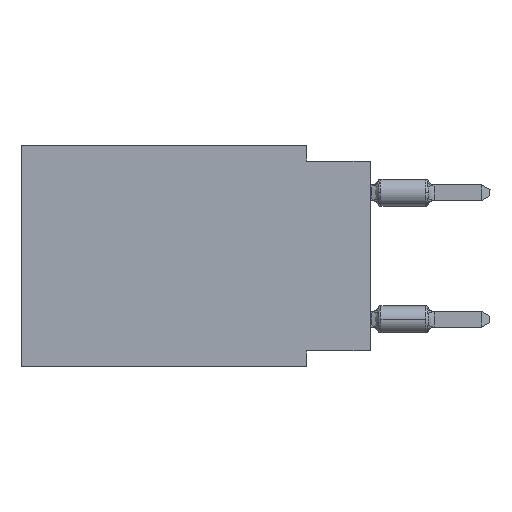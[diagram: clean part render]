
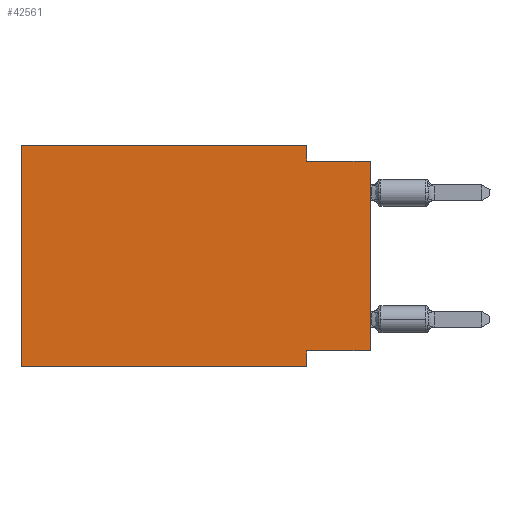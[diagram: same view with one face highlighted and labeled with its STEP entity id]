
A CAD part, left-side view. The second image highlights one B-rep face of the part: STEP entity #42561.
In plain terms, the highlighted planar face has unit normal (-1, 0, 0).
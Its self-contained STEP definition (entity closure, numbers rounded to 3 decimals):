
#1793 = VERTEX_POINT ( 'NONE', #42970 ) ;
#2512 = CARTESIAN_POINT ( 'NONE',  ( 0., 13.97, 0. ) ) ;
#2854 = VECTOR ( 'NONE', #18139, 1000. ) ;
#2898 = CARTESIAN_POINT ( 'NONE',  ( 0., 0., -8.255 ) ) ;
#2917 = EDGE_CURVE ( 'NONE', #43926, #25107, #45139, .T. ) ;
#3358 = CARTESIAN_POINT ( 'NONE',  ( 0., 2.54, 0. ) ) ;
#3403 = CARTESIAN_POINT ( 'NONE',  ( 0., 2.54, -8.89 ) ) ;
#4902 = EDGE_CURVE ( 'NONE', #26512, #8905, #33736, .T. ) ;
#6774 = CARTESIAN_POINT ( 'NONE',  ( 0., 0., -0.635 ) ) ;
#7037 = ORIENTED_EDGE ( 'NONE', *, *, #20022, .F. ) ;
#7201 = LINE ( 'NONE', #2512, #2854 ) ;
#8905 = VERTEX_POINT ( 'NONE', #49369 ) ;
#9450 = CARTESIAN_POINT ( 'NONE',  ( 0., 2.54, 0. ) ) ;
#10574 = LINE ( 'NONE', #26464, #40328 ) ;
#11358 = DIRECTION ( 'NONE',  ( 0., 0., -1. ) ) ;
#11938 = CARTESIAN_POINT ( 'NONE',  ( 0., 0., -0.635 ) ) ;
#12310 = ORIENTED_EDGE ( 'NONE', *, *, #32414, .T. ) ;
#12445 = LINE ( 'NONE', #11938, #13998 ) ;
#13086 = CARTESIAN_POINT ( 'NONE',  ( 0., 13.97, -8.89 ) ) ;
#13496 = VECTOR ( 'NONE', #34929, 1000. ) ;
#13998 = VECTOR ( 'NONE', #31977, 1000. ) ;
#14759 = EDGE_CURVE ( 'NONE', #8905, #43926, #7201, .T. ) ;
#14788 = VECTOR ( 'NONE', #29049, 1000. ) ;
#15261 = FACE_OUTER_BOUND ( 'NONE', #15369, .T. ) ;
#15296 = LINE ( 'NONE', #38744, #50191 ) ;
#15317 = ORIENTED_EDGE ( 'NONE', *, *, #14759, .F. ) ;
#15369 = EDGE_LOOP ( 'NONE', ( #43587, #40888, #17756, #15317, #21226, #12310, #7037, #40070 ) ) ;
#15669 = CARTESIAN_POINT ( 'NONE',  ( 0., 13.97, -8.89 ) ) ;
#17756 = ORIENTED_EDGE ( 'NONE', *, *, #2917, .F. ) ;
#17856 = CARTESIAN_POINT ( 'NONE',  ( 0., 13.97, 0. ) ) ;
#18139 = DIRECTION ( 'NONE',  ( 0., -1., 0. ) ) ;
#19164 = VECTOR ( 'NONE', #30226, 1000. ) ;
#19426 = PLANE ( 'NONE',  #29995 ) ;
#19574 = LINE ( 'NONE', #15669, #13496 ) ;
#20022 = EDGE_CURVE ( 'NONE', #1793, #25607, #10574, .T. ) ;
#21226 = ORIENTED_EDGE ( 'NONE', *, *, #4902, .F. ) ;
#21905 = LINE ( 'NONE', #2898, #19164 ) ;
#24367 = VERTEX_POINT ( 'NONE', #6774 ) ;
#25107 = VERTEX_POINT ( 'NONE', #42843 ) ;
#25341 = DIRECTION ( 'NONE',  ( 0., 0., -1. ) ) ;
#25607 = VERTEX_POINT ( 'NONE', #3403 ) ;
#26464 = CARTESIAN_POINT ( 'NONE',  ( 0., 2.54, -8.89 ) ) ;
#26512 = VERTEX_POINT ( 'NONE', #13086 ) ;
#28663 = EDGE_CURVE ( 'NONE', #25107, #24367, #12445, .T. ) ;
#29049 = DIRECTION ( 'NONE',  ( 0., 0., 1. ) ) ;
#29995 = AXIS2_PLACEMENT_3D ( 'NONE', #31129, #33819, #11358 ) ;
#30226 = DIRECTION ( 'NONE',  ( 0., 1., 0. ) ) ;
#31129 = CARTESIAN_POINT ( 'NONE',  ( 0., 13.97, 0. ) ) ;
#31977 = DIRECTION ( 'NONE',  ( 0., -1., 0. ) ) ;
#32414 = EDGE_CURVE ( 'NONE', #26512, #25607, #19574, .T. ) ;
#33736 = LINE ( 'NONE', #17856, #14788 ) ;
#33819 = DIRECTION ( 'NONE',  ( 1., 0., 0. ) ) ;
#34573 = DIRECTION ( 'NONE',  ( 0., 0., 1. ) ) ;
#34929 = DIRECTION ( 'NONE',  ( 0., -1., 0. ) ) ;
#38744 = CARTESIAN_POINT ( 'NONE',  ( 0., 0., 0. ) ) ;
#39744 = CARTESIAN_POINT ( 'NONE',  ( 0., 0., -8.255 ) ) ;
#40070 = ORIENTED_EDGE ( 'NONE', *, *, #42115, .F. ) ;
#40328 = VECTOR ( 'NONE', #42878, 1000. ) ;
#40888 = ORIENTED_EDGE ( 'NONE', *, *, #28663, .F. ) ;
#42115 = EDGE_CURVE ( 'NONE', #44350, #1793, #21905, .T. ) ;
#42561 = ADVANCED_FACE ( 'NONE', ( #15261 ), #19426, .F. ) ;
#42843 = CARTESIAN_POINT ( 'NONE',  ( 0., 2.54, -0.635 ) ) ;
#42878 = DIRECTION ( 'NONE',  ( 0., 0., -1. ) ) ;
#42970 = CARTESIAN_POINT ( 'NONE',  ( 0., 2.54, -8.255 ) ) ;
#43587 = ORIENTED_EDGE ( 'NONE', *, *, #45376, .T. ) ;
#43926 = VERTEX_POINT ( 'NONE', #3358 ) ;
#44350 = VERTEX_POINT ( 'NONE', #39744 ) ;
#45139 = LINE ( 'NONE', #9450, #49946 ) ;
#45376 = EDGE_CURVE ( 'NONE', #44350, #24367, #15296, .T. ) ;
#49369 = CARTESIAN_POINT ( 'NONE',  ( 0., 13.97, 0. ) ) ;
#49946 = VECTOR ( 'NONE', #25341, 1000. ) ;
#50191 = VECTOR ( 'NONE', #34573, 1000. ) ;
